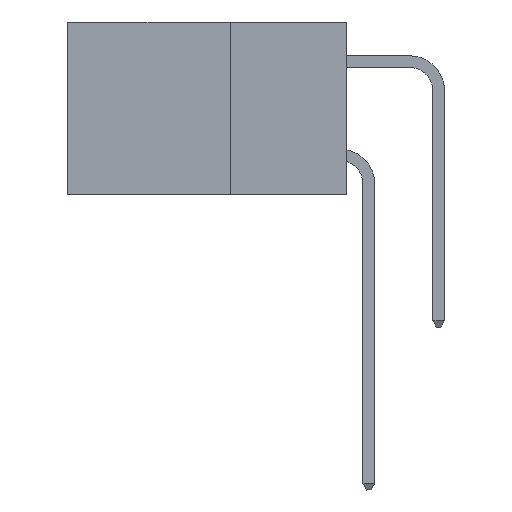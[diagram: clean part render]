
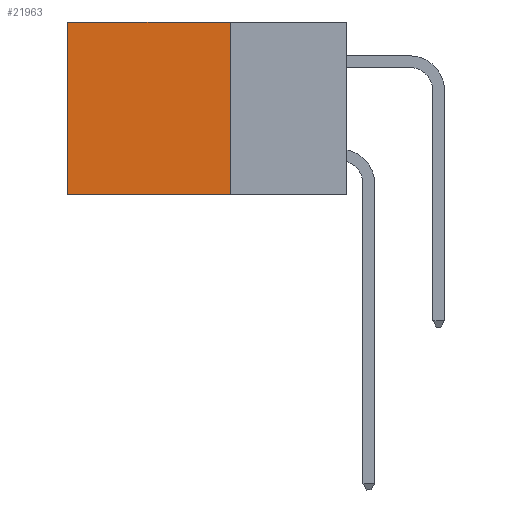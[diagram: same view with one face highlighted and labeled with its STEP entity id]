
A CAD part, left-side view. The second image highlights one B-rep face of the part: STEP entity #21963.
In plain terms, the highlighted planar face has unit normal (-1, 0, 0).
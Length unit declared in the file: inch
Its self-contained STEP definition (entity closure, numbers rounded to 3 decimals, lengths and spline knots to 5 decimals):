
#46 = LINE ( 'NONE', #22071, #18770 ) ;
#374 = EDGE_CURVE ( 'NONE', #15545, #11928, #7602, .T. ) ;
#797 = AXIS2_PLACEMENT_3D ( 'NONE', #8248, #21030, #10152 ) ;
#822 = CARTESIAN_POINT ( 'NONE',  ( 0.2875, 0.6, 0. ) ) ;
#2232 = CARTESIAN_POINT ( 'NONE',  ( 0.2875, 0.25, 0. ) ) ;
#4297 = DIRECTION ( 'NONE',  ( 0., 1., 0. ) ) ;
#4620 = ORIENTED_EDGE ( 'NONE', *, *, #7818, .T. ) ;
#4624 = LINE ( 'NONE', #822, #13475 ) ;
#5586 = EDGE_LOOP ( 'NONE', ( #20927, #10749, #20537, #4620 ) ) ;
#6318 = FACE_OUTER_BOUND ( 'NONE', #5586, .T. ) ;
#7602 = LINE ( 'NONE', #13341, #12434 ) ;
#7818 = EDGE_CURVE ( 'NONE', #13997, #15655, #46, .T. ) ;
#8248 = CARTESIAN_POINT ( 'NONE',  ( 0.2875, 0.25, 0. ) ) ;
#9364 = DIRECTION ( 'NONE',  ( 0., 1., 0. ) ) ;
#10152 = DIRECTION ( 'NONE',  ( 0., 0., -1. ) ) ;
#10371 = EDGE_CURVE ( 'NONE', #13997, #15545, #12137, .T. ) ;
#10680 = CARTESIAN_POINT ( 'NONE',  ( 0.2875, 0.6, 0. ) ) ;
#10749 = ORIENTED_EDGE ( 'NONE', *, *, #374, .F. ) ;
#11928 = VERTEX_POINT ( 'NONE', #16531 ) ;
#12137 = LINE ( 'NONE', #19343, #20637 ) ;
#12434 = VECTOR ( 'NONE', #4297, 39.37008 ) ;
#13341 = CARTESIAN_POINT ( 'NONE',  ( 0.2875, 0.25, -0.37 ) ) ;
#13475 = VECTOR ( 'NONE', #13513, 39.37008 ) ;
#13513 = DIRECTION ( 'NONE',  ( 0., 0., -1. ) ) ;
#13997 = VERTEX_POINT ( 'NONE', #2232 ) ;
#15545 = VERTEX_POINT ( 'NONE', #15553 ) ;
#15553 = CARTESIAN_POINT ( 'NONE',  ( 0.2875, 0.25, -0.37 ) ) ;
#15601 = PLANE ( 'NONE',  #797 ) ;
#15655 = VERTEX_POINT ( 'NONE', #10680 ) ;
#16531 = CARTESIAN_POINT ( 'NONE',  ( 0.2875, 0.6, -0.37 ) ) ;
#18770 = VECTOR ( 'NONE', #9364, 39.37008 ) ;
#19311 = EDGE_CURVE ( 'NONE', #15655, #11928, #4624, .T. ) ;
#19343 = CARTESIAN_POINT ( 'NONE',  ( 0.2875, 0.25, 0. ) ) ;
#19425 = DIRECTION ( 'NONE',  ( 0., 0., -1. ) ) ;
#20537 = ORIENTED_EDGE ( 'NONE', *, *, #10371, .F. ) ;
#20637 = VECTOR ( 'NONE', #19425, 39.37008 ) ;
#20927 = ORIENTED_EDGE ( 'NONE', *, *, #19311, .T. ) ;
#21030 = DIRECTION ( 'NONE',  ( 1., 0., 0. ) ) ;
#21963 = ADVANCED_FACE ( 'NONE', ( #6318 ), #15601, .F. ) ;
#22071 = CARTESIAN_POINT ( 'NONE',  ( 0.2875, 0.25, 0. ) ) ;
